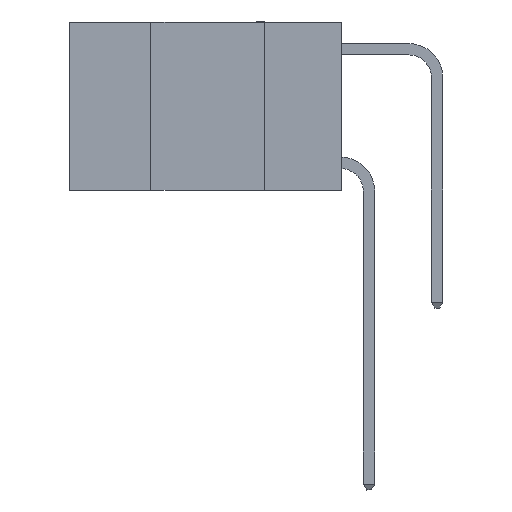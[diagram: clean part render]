
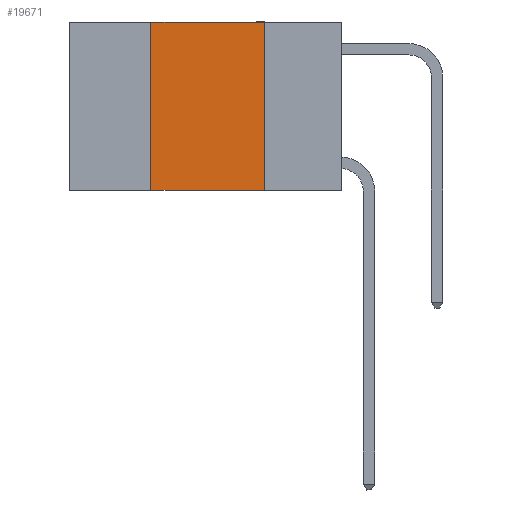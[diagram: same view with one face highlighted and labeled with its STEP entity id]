
A CAD part, left-side view. The second image highlights one B-rep face of the part: STEP entity #19671.
In plain terms, the highlighted planar face has unit normal (-1, 0, 0).
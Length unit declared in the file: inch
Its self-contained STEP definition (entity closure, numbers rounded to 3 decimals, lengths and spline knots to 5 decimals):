
#1024 = EDGE_CURVE ( 'NONE', #6709, #7247, #7362, .T. ) ;
#1109 = EDGE_CURVE ( 'NONE', #12646, #6709, #22578, .T. ) ;
#1244 = CARTESIAN_POINT ( 'NONE',  ( 0., 0.6, 0. ) ) ;
#1547 = EDGE_LOOP ( 'NONE', ( #17627, #18343, #7039, #1636 ) ) ;
#1636 = ORIENTED_EDGE ( 'NONE', *, *, #16832, .T. ) ;
#3087 = CARTESIAN_POINT ( 'NONE',  ( 0., 0.42, 0. ) ) ;
#3567 = CARTESIAN_POINT ( 'NONE',  ( 0., 0.6, 0. ) ) ;
#4822 = AXIS2_PLACEMENT_3D ( 'NONE', #1244, #8200, #23995 ) ;
#5523 = DIRECTION ( 'NONE',  ( 0., 0., 1. ) ) ;
#5647 = VECTOR ( 'NONE', #5523, 39.37008 ) ;
#5860 = DIRECTION ( 'NONE',  ( 0., -1., 0. ) ) ;
#6709 = VERTEX_POINT ( 'NONE', #19893 ) ;
#7039 = ORIENTED_EDGE ( 'NONE', *, *, #7181, .F. ) ;
#7181 = EDGE_CURVE ( 'NONE', #12120, #12646, #11678, .T. ) ;
#7247 = VERTEX_POINT ( 'NONE', #14737 ) ;
#7362 = LINE ( 'NONE', #14590, #19400 ) ;
#8200 = DIRECTION ( 'NONE',  ( 1., 0., 0. ) ) ;
#10555 = VECTOR ( 'NONE', #5860, 39.37008 ) ;
#11678 = LINE ( 'NONE', #14549, #5647 ) ;
#12120 = VERTEX_POINT ( 'NONE', #21652 ) ;
#12646 = VERTEX_POINT ( 'NONE', #3087 ) ;
#14549 = CARTESIAN_POINT ( 'NONE',  ( 0., 0.42, 0. ) ) ;
#14590 = CARTESIAN_POINT ( 'NONE',  ( 0., 0.17, 0. ) ) ;
#14737 = CARTESIAN_POINT ( 'NONE',  ( 0., 0.17, -0.37 ) ) ;
#16832 = EDGE_CURVE ( 'NONE', #12120, #7247, #20638, .T. ) ;
#16838 = DIRECTION ( 'NONE',  ( 0., 0., -1. ) ) ;
#17627 = ORIENTED_EDGE ( 'NONE', *, *, #1024, .F. ) ;
#18343 = ORIENTED_EDGE ( 'NONE', *, *, #1109, .F. ) ;
#19400 = VECTOR ( 'NONE', #16838, 39.37008 ) ;
#19671 = ADVANCED_FACE ( 'NONE', ( #25278 ), #21719, .F. ) ;
#19893 = CARTESIAN_POINT ( 'NONE',  ( 0., 0.17, 0. ) ) ;
#20638 = LINE ( 'NONE', #21457, #28873 ) ;
#21457 = CARTESIAN_POINT ( 'NONE',  ( 0., 0.6, -0.37 ) ) ;
#21652 = CARTESIAN_POINT ( 'NONE',  ( 0., 0.42, -0.37 ) ) ;
#21719 = PLANE ( 'NONE',  #4822 ) ;
#22578 = LINE ( 'NONE', #3567, #10555 ) ;
#23767 = DIRECTION ( 'NONE',  ( 0., -1., 0. ) ) ;
#23995 = DIRECTION ( 'NONE',  ( 0., 0., -1. ) ) ;
#25278 = FACE_OUTER_BOUND ( 'NONE', #1547, .T. ) ;
#28873 = VECTOR ( 'NONE', #23767, 39.37008 ) ;
